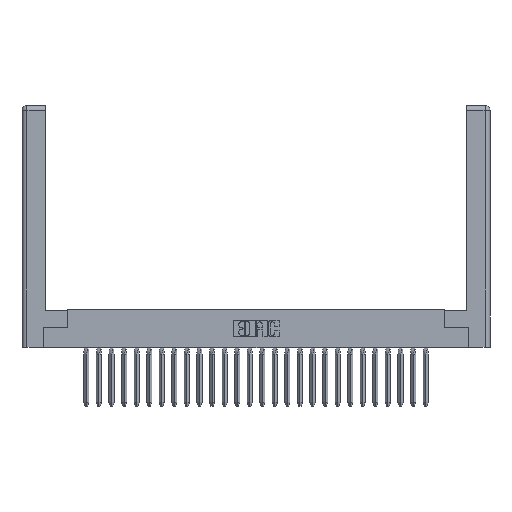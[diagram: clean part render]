
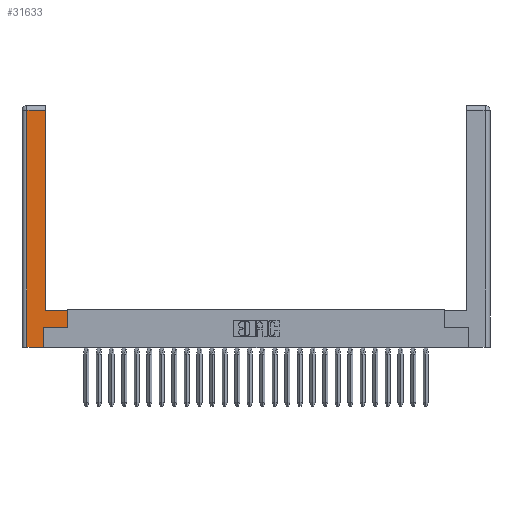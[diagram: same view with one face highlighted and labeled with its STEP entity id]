
A CAD part, top view. The second image highlights one B-rep face of the part: STEP entity #31633.
In plain terms, the highlighted planar face has unit normal (0, 0, 1).
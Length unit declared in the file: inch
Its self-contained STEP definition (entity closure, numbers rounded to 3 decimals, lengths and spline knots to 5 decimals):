
#540 = VECTOR ( 'NONE', #48764, 39.37008 ) ;
#880 = EDGE_CURVE ( 'NONE', #20413, #34725, #4979, .T. ) ;
#1478 = LINE ( 'NONE', #2549, #42468 ) ;
#2040 = CARTESIAN_POINT ( 'NONE',  ( 0.0615, 2.94, 0. ) ) ;
#2146 = VERTEX_POINT ( 'NONE', #35828 ) ;
#2549 = CARTESIAN_POINT ( 'NONE',  ( 0.295, 3., 0. ) ) ;
#2791 = EDGE_CURVE ( 'NONE', #55468, #20413, #8986, .T. ) ;
#4190 = CARTESIAN_POINT ( 'NONE',  ( 0.265, 0.245, 0. ) ) ;
#4979 = LINE ( 'NONE', #4190, #32484 ) ;
#5244 = ORIENTED_EDGE ( 'NONE', *, *, #2791, .T. ) ;
#5949 = CARTESIAN_POINT ( 'NONE',  ( 0.0615, 0., 0. ) ) ;
#7490 = LINE ( 'NONE', #24005, #13802 ) ;
#8986 = LINE ( 'NONE', #20318, #16030 ) ;
#9136 = ORIENTED_EDGE ( 'NONE', *, *, #44237, .T. ) ;
#9974 = VERTEX_POINT ( 'NONE', #44207 ) ;
#10232 = CARTESIAN_POINT ( 'NONE',  ( 0.0615, 2.94, 0. ) ) ;
#12449 = LINE ( 'NONE', #2040, #17418 ) ;
#13108 = CARTESIAN_POINT ( 'NONE',  ( 0.565, 0.245, 0. ) ) ;
#13186 = ORIENTED_EDGE ( 'NONE', *, *, #47691, .T. ) ;
#13802 = VECTOR ( 'NONE', #15122, 39.37008 ) ;
#15117 = DIRECTION ( 'NONE',  ( -1., 0., 0. ) ) ;
#15122 = DIRECTION ( 'NONE',  ( 0., 1., 0. ) ) ;
#15486 = PLANE ( 'NONE',  #24469 ) ;
#15896 = DIRECTION ( 'NONE',  ( 0., 0., -1. ) ) ;
#16030 = VECTOR ( 'NONE', #33752, 39.37008 ) ;
#16070 = CARTESIAN_POINT ( 'NONE',  ( 0.265, 0.245, 0. ) ) ;
#17316 = VERTEX_POINT ( 'NONE', #20026 ) ;
#17378 = ORIENTED_EDGE ( 'NONE', *, *, #28141, .T. ) ;
#17418 = VECTOR ( 'NONE', #57194, 39.37008 ) ;
#19430 = EDGE_CURVE ( 'NONE', #49715, #55468, #54560, .T. ) ;
#20026 = CARTESIAN_POINT ( 'NONE',  ( 0.565, 0.45, 0. ) ) ;
#20318 = CARTESIAN_POINT ( 'NONE',  ( 0.265, 0., 0. ) ) ;
#20337 = LINE ( 'NONE', #13108, #540 ) ;
#20358 = VERTEX_POINT ( 'NONE', #24104 ) ;
#20413 = VERTEX_POINT ( 'NONE', #34387 ) ;
#20910 = EDGE_CURVE ( 'NONE', #34725, #20358, #20337, .T. ) ;
#24005 = CARTESIAN_POINT ( 'NONE',  ( 0.565, 0.45, 0. ) ) ;
#24104 = CARTESIAN_POINT ( 'NONE',  ( 0.565, 0.245, 0. ) ) ;
#24469 = AXIS2_PLACEMENT_3D ( 'NONE', #47154, #15896, #38844 ) ;
#24566 = LINE ( 'NONE', #37475, #33071 ) ;
#28141 = EDGE_CURVE ( 'NONE', #20358, #17316, #7490, .T. ) ;
#28276 = VECTOR ( 'NONE', #56491, 39.37008 ) ;
#29368 = DIRECTION ( 'NONE',  ( 0., 1., 0. ) ) ;
#29574 = FACE_OUTER_BOUND ( 'NONE', #50634, .T. ) ;
#31633 = ADVANCED_FACE ( 'NONE', ( #29574 ), #15486, .F. ) ;
#32484 = VECTOR ( 'NONE', #52405, 39.37008 ) ;
#33071 = VECTOR ( 'NONE', #15117, 39.37008 ) ;
#33718 = CARTESIAN_POINT ( 'NONE',  ( 0.0615, 0., 0. ) ) ;
#33752 = DIRECTION ( 'NONE',  ( 1., 0., 0. ) ) ;
#34387 = CARTESIAN_POINT ( 'NONE',  ( 0.265, 0., 0. ) ) ;
#34725 = VERTEX_POINT ( 'NONE', #16070 ) ;
#35828 = CARTESIAN_POINT ( 'NONE',  ( 0.295, 2.94, 0. ) ) ;
#37475 = CARTESIAN_POINT ( 'NONE',  ( 0.295, 0.45, 0. ) ) ;
#38844 = DIRECTION ( 'NONE',  ( -1., 0., 0. ) ) ;
#39884 = EDGE_CURVE ( 'NONE', #2146, #49715, #12449, .T. ) ;
#42468 = VECTOR ( 'NONE', #29368, 39.37008 ) ;
#44207 = CARTESIAN_POINT ( 'NONE',  ( 0.295, 0.45, 0. ) ) ;
#44237 = EDGE_CURVE ( 'NONE', #17316, #9974, #24566, .T. ) ;
#45530 = ORIENTED_EDGE ( 'NONE', *, *, #39884, .T. ) ;
#46709 = ORIENTED_EDGE ( 'NONE', *, *, #20910, .T. ) ;
#46938 = ORIENTED_EDGE ( 'NONE', *, *, #19430, .T. ) ;
#47154 = CARTESIAN_POINT ( 'NONE',  ( 0., 0., 0. ) ) ;
#47691 = EDGE_CURVE ( 'NONE', #9974, #2146, #1478, .T. ) ;
#48764 = DIRECTION ( 'NONE',  ( 1., 0., 0. ) ) ;
#49715 = VERTEX_POINT ( 'NONE', #10232 ) ;
#50634 = EDGE_LOOP ( 'NONE', ( #13186, #45530, #46938, #5244, #57048, #46709, #17378, #9136 ) ) ;
#52405 = DIRECTION ( 'NONE',  ( 0., 1., 0. ) ) ;
#54560 = LINE ( 'NONE', #33718, #28276 ) ;
#55468 = VERTEX_POINT ( 'NONE', #5949 ) ;
#56491 = DIRECTION ( 'NONE',  ( 0., -1., 0. ) ) ;
#57048 = ORIENTED_EDGE ( 'NONE', *, *, #880, .T. ) ;
#57194 = DIRECTION ( 'NONE',  ( -1., 0., 0. ) ) ;
